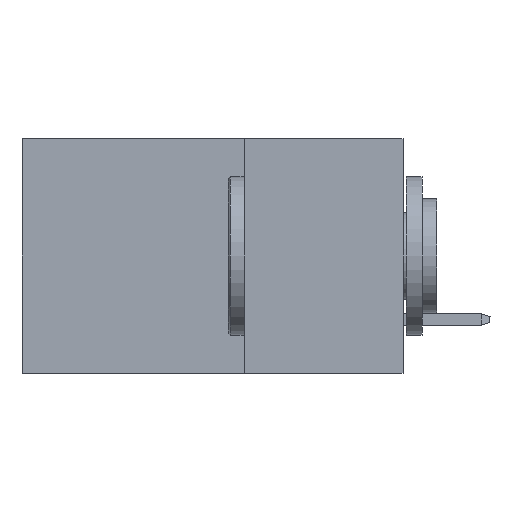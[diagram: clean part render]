
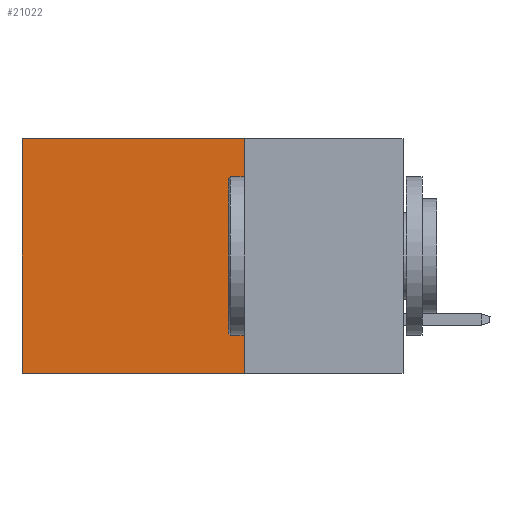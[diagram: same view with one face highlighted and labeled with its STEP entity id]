
A CAD part, left-side view. The second image highlights one B-rep face of the part: STEP entity #21022.
In plain terms, the highlighted planar face has unit normal (-1, 0, 0).
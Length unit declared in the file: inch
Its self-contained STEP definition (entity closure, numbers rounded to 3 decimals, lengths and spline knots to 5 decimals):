
#39 = VECTOR ( 'NONE', #13650, 39.37008 ) ;
#356 = VERTEX_POINT ( 'NONE', #7771 ) ;
#3180 = EDGE_LOOP ( 'NONE', ( #39010, #25507, #15504, #34372 ) ) ;
#3499 = CARTESIAN_POINT ( 'NONE',  ( 0.2875, 0.25, 0. ) ) ;
#5334 = VERTEX_POINT ( 'NONE', #40606 ) ;
#5368 = DIRECTION ( 'NONE',  ( 0., 0., -1. ) ) ;
#5799 = LINE ( 'NONE', #6236, #39706 ) ;
#6236 = CARTESIAN_POINT ( 'NONE',  ( 0.2875, 0.6, 0. ) ) ;
#7017 = DIRECTION ( 'NONE',  ( 0., 0., -1. ) ) ;
#7771 = CARTESIAN_POINT ( 'NONE',  ( 0.2875, 0.6, 0. ) ) ;
#9593 = LINE ( 'NONE', #3499, #19715 ) ;
#9901 = VERTEX_POINT ( 'NONE', #42071 ) ;
#9957 = LINE ( 'NONE', #30750, #39 ) ;
#10263 = CARTESIAN_POINT ( 'NONE',  ( 0.2875, 0.25, 0. ) ) ;
#11721 = EDGE_CURVE ( 'NONE', #9901, #356, #9957, .T. ) ;
#13650 = DIRECTION ( 'NONE',  ( 0., 1., 0. ) ) ;
#14788 = LINE ( 'NONE', #31694, #20828 ) ;
#15504 = ORIENTED_EDGE ( 'NONE', *, *, #25584, .F. ) ;
#18466 = DIRECTION ( 'NONE',  ( 0., 1., 0. ) ) ;
#19616 = PLANE ( 'NONE',  #22897 ) ;
#19715 = VECTOR ( 'NONE', #42743, 39.37008 ) ;
#20828 = VECTOR ( 'NONE', #18466, 39.37008 ) ;
#21022 = ADVANCED_FACE ( 'NONE', ( #39941 ), #19616, .F. ) ;
#21304 = EDGE_CURVE ( 'NONE', #42553, #5334, #14788, .T. ) ;
#22897 = AXIS2_PLACEMENT_3D ( 'NONE', #10263, #39523, #7017 ) ;
#25507 = ORIENTED_EDGE ( 'NONE', *, *, #21304, .F. ) ;
#25584 = EDGE_CURVE ( 'NONE', #9901, #42553, #9593, .T. ) ;
#27332 = CARTESIAN_POINT ( 'NONE',  ( 0.2875, 0.25, -0.37 ) ) ;
#30750 = CARTESIAN_POINT ( 'NONE',  ( 0.2875, 0.25, 0. ) ) ;
#31694 = CARTESIAN_POINT ( 'NONE',  ( 0.2875, 0.25, -0.37 ) ) ;
#32481 = EDGE_CURVE ( 'NONE', #356, #5334, #5799, .T. ) ;
#34372 = ORIENTED_EDGE ( 'NONE', *, *, #11721, .T. ) ;
#39010 = ORIENTED_EDGE ( 'NONE', *, *, #32481, .T. ) ;
#39523 = DIRECTION ( 'NONE',  ( 1., 0., 0. ) ) ;
#39706 = VECTOR ( 'NONE', #5368, 39.37008 ) ;
#39941 = FACE_OUTER_BOUND ( 'NONE', #3180, .T. ) ;
#40606 = CARTESIAN_POINT ( 'NONE',  ( 0.2875, 0.6, -0.37 ) ) ;
#42071 = CARTESIAN_POINT ( 'NONE',  ( 0.2875, 0.25, 0. ) ) ;
#42553 = VERTEX_POINT ( 'NONE', #27332 ) ;
#42743 = DIRECTION ( 'NONE',  ( 0., 0., -1. ) ) ;
